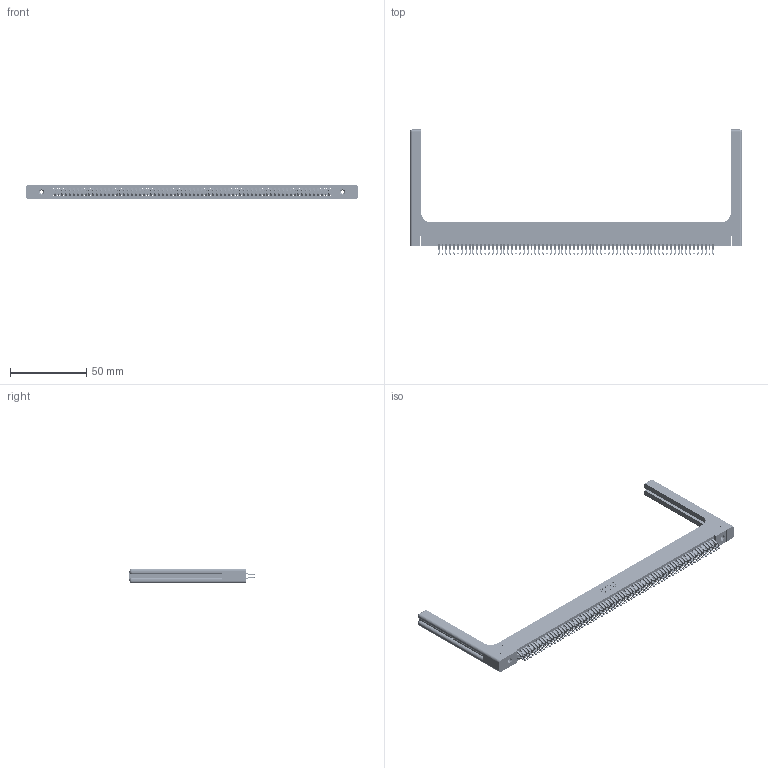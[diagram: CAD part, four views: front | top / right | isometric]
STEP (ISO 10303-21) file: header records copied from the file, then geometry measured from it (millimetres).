
FILE_DESCRIPTION (( 'STEP AP203' ), '1' );
FILE_NAME ('395-144-555-258.STEP', '2019-10-30T16:29:04', ( '' ), ( '' ), 'SwSTEP 2.0', 'SolidWorks 2016', '' );
FILE_SCHEMA (( 'CONFIG_CONTROL_DESIGN' ));
Length unit declared in the file: inch
Products named in the file (5): 395-144-555-258; 345 Part_Flush Mounting Lugs - 0.156 Dia-TH; 345-292-001_555 Tail; 345-250-001_345-250-001-102; 345-220-058_345-220-058
Assembly tree (149 placements, depth 2):
  395-144-555-258
    345 Part_Flush Mounting Lugs - 0.156 Dia-TH
    345-292-001_555 Tail  x144
    345-250-001_345-250-001-102  x2
    345-220-058_345-220-058  x2
Bounding box: 217.91 x 82.09 x 9.4 mm (x, y, z)
Volume: 30338.9 mm3; surface area: 39411 mm2
Topology: 149 solids, 149 shells, 8446 faces, 26495 edges, 17642 vertices
Faces by surface type: plane 4692, cylinder 3694, bspline 36, cone 12, sphere 8, torus 4
Entity records: 57962 total; most frequent: CARTESIAN_POINT 10715, ORIENTED_EDGE 9416, DIRECTION 8312, EDGE_CURVE 4708, VECTOR 4176, LINE 4176, VERTEX_POINT 3130, AXIS2_PLACEMENT_3D 2068
